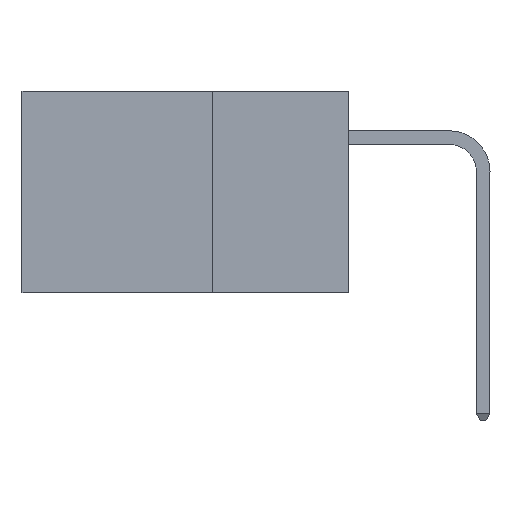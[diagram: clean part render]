
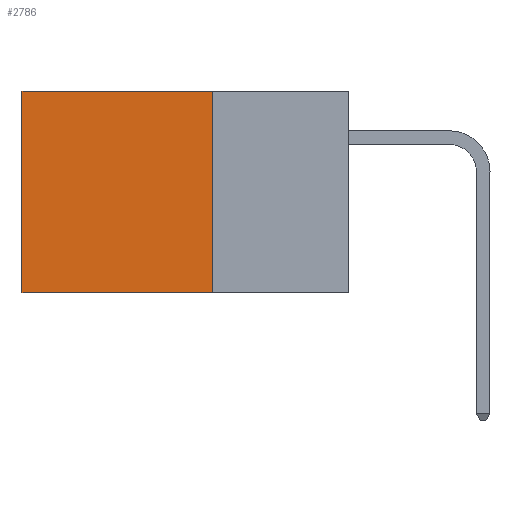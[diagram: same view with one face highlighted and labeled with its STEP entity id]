
A CAD part, left-side view. The second image highlights one B-rep face of the part: STEP entity #2786.
In plain terms, the highlighted planar face has unit normal (-1, 0, 0).
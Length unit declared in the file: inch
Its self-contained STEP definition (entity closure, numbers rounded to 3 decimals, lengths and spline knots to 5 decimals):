
#372 = EDGE_CURVE ( 'NONE', #7027, #4089, #8781, .T. ) ;
#465 = VERTEX_POINT ( 'NONE', #12440 ) ;
#698 = DIRECTION ( 'NONE',  ( 0., 1., 0. ) ) ;
#851 = CARTESIAN_POINT ( 'NONE',  ( 0.2875, 0.6, 0. ) ) ;
#881 = PLANE ( 'NONE',  #3499 ) ;
#1500 = LINE ( 'NONE', #13380, #2196 ) ;
#1917 = DIRECTION ( 'NONE',  ( 1., 0., 0. ) ) ;
#2196 = VECTOR ( 'NONE', #698, 39.37008 ) ;
#2244 = DIRECTION ( 'NONE',  ( 0., 0., -1. ) ) ;
#2786 = ADVANCED_FACE ( 'NONE', ( #3086 ), #881, .F. ) ;
#3027 = CARTESIAN_POINT ( 'NONE',  ( 0.2875, 0.25, 0. ) ) ;
#3070 = CARTESIAN_POINT ( 'NONE',  ( 0.2875, 0.25, 0. ) ) ;
#3086 = FACE_OUTER_BOUND ( 'NONE', #4629, .T. ) ;
#3499 = AXIS2_PLACEMENT_3D ( 'NONE', #3027, #1917, #9406 ) ;
#3642 = VERTEX_POINT ( 'NONE', #851 ) ;
#4089 = VERTEX_POINT ( 'NONE', #11826 ) ;
#4604 = CARTESIAN_POINT ( 'NONE',  ( 0.2875, 0.25, -0.37 ) ) ;
#4629 = EDGE_LOOP ( 'NONE', ( #7607, #8334, #4937, #12307 ) ) ;
#4937 = ORIENTED_EDGE ( 'NONE', *, *, #372, .F. ) ;
#4943 = LINE ( 'NONE', #5318, #7767 ) ;
#5318 = CARTESIAN_POINT ( 'NONE',  ( 0.2875, 0.6, 0. ) ) ;
#6812 = CARTESIAN_POINT ( 'NONE',  ( 0.2875, 0.25, 0. ) ) ;
#6904 = DIRECTION ( 'NONE',  ( 0., 0., -1. ) ) ;
#6943 = VECTOR ( 'NONE', #6904, 39.37008 ) ;
#7027 = VERTEX_POINT ( 'NONE', #3070 ) ;
#7607 = ORIENTED_EDGE ( 'NONE', *, *, #12951, .T. ) ;
#7767 = VECTOR ( 'NONE', #2244, 39.37008 ) ;
#8334 = ORIENTED_EDGE ( 'NONE', *, *, #11426, .F. ) ;
#8781 = LINE ( 'NONE', #6812, #6943 ) ;
#9232 = VECTOR ( 'NONE', #13215, 39.37008 ) ;
#9406 = DIRECTION ( 'NONE',  ( 0., 0., -1. ) ) ;
#11426 = EDGE_CURVE ( 'NONE', #4089, #465, #12712, .T. ) ;
#11826 = CARTESIAN_POINT ( 'NONE',  ( 0.2875, 0.25, -0.37 ) ) ;
#12265 = EDGE_CURVE ( 'NONE', #7027, #3642, #1500, .T. ) ;
#12307 = ORIENTED_EDGE ( 'NONE', *, *, #12265, .T. ) ;
#12440 = CARTESIAN_POINT ( 'NONE',  ( 0.2875, 0.6, -0.37 ) ) ;
#12712 = LINE ( 'NONE', #4604, #9232 ) ;
#12951 = EDGE_CURVE ( 'NONE', #3642, #465, #4943, .T. ) ;
#13215 = DIRECTION ( 'NONE',  ( 0., 1., 0. ) ) ;
#13380 = CARTESIAN_POINT ( 'NONE',  ( 0.2875, 0.25, 0. ) ) ;
